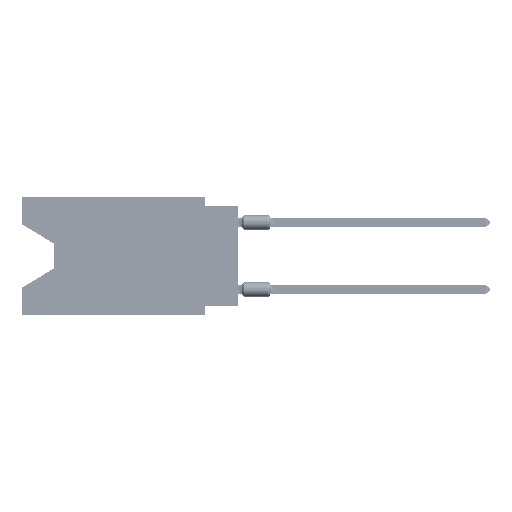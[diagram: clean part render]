
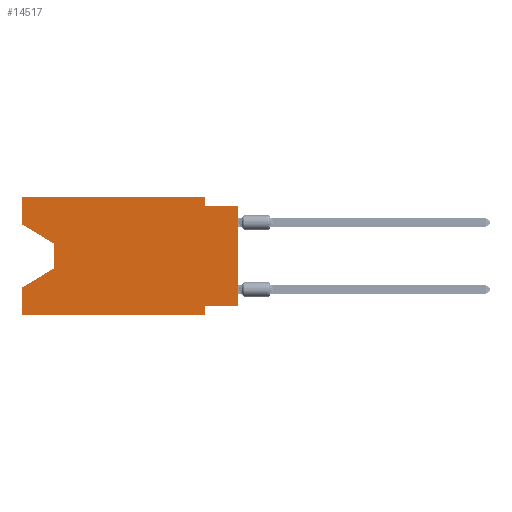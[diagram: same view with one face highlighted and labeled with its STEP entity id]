
A CAD part, left-side view. The second image highlights one B-rep face of the part: STEP entity #14517.
In plain terms, the highlighted planar face has unit normal (-1, 0, 0).
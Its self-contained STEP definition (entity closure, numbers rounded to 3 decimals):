
#1464 = EDGE_LOOP ( 'NONE', ( #14148, #25218, #67241, #67048, #18432, #14422, #58843, #45824, #65367, #66566, #65498, #14328 ) ) ;
#2591 = DIRECTION ( 'NONE',  ( 0., -1., 0. ) ) ;
#3326 = CARTESIAN_POINT ( 'NONE',  ( 0., 16.383, -6.852 ) ) ;
#5219 = VECTOR ( 'NONE', #29691, 1000. ) ;
#6168 = CARTESIAN_POINT ( 'NONE',  ( 0., 16.383, 0. ) ) ;
#6570 = CARTESIAN_POINT ( 'NONE',  ( 0., 13.97, -3.505 ) ) ;
#6710 = CARTESIAN_POINT ( 'NONE',  ( 0., 16.383, 0. ) ) ;
#7194 = DIRECTION ( 'NONE',  ( 0., -0.855, -0.519 ) ) ;
#7883 = CARTESIAN_POINT ( 'NONE',  ( 0., 16.383, -2.038 ) ) ;
#8289 = DIRECTION ( 'NONE',  ( 0., 0.855, -0.519 ) ) ;
#8771 = DIRECTION ( 'NONE',  ( 0., -1., 0. ) ) ;
#8777 = CARTESIAN_POINT ( 'NONE',  ( 0., 13.97, -3.505 ) ) ;
#9254 = CARTESIAN_POINT ( 'NONE',  ( 0., 2.54, -8.89 ) ) ;
#11705 = VECTOR ( 'NONE', #17852, 1000. ) ;
#11786 = CARTESIAN_POINT ( 'NONE',  ( 0., 2.54, 0. ) ) ;
#11862 = EDGE_CURVE ( 'NONE', #12898, #56876, #51616, .T. ) ;
#12177 = DIRECTION ( 'NONE',  ( 0., 0., -1. ) ) ;
#12898 = VERTEX_POINT ( 'NONE', #27450 ) ;
#13046 = CARTESIAN_POINT ( 'NONE',  ( 0., 0., -0.635 ) ) ;
#13644 = VERTEX_POINT ( 'NONE', #22750 ) ;
#14148 = ORIENTED_EDGE ( 'NONE', *, *, #18397, .T. ) ;
#14284 = LINE ( 'NONE', #56065, #5219 ) ;
#14328 = ORIENTED_EDGE ( 'NONE', *, *, #14355, .F. ) ;
#14355 = EDGE_CURVE ( 'NONE', #37788, #39389, #25358, .T. ) ;
#14422 = ORIENTED_EDGE ( 'NONE', *, *, #33079, .F. ) ;
#14517 = ADVANCED_FACE ( 'NONE', ( #53074 ), #16778, .F. ) ;
#15247 = CARTESIAN_POINT ( 'NONE',  ( 0., 16.383, -8.89 ) ) ;
#16778 = PLANE ( 'NONE',  #20786 ) ;
#17025 = VERTEX_POINT ( 'NONE', #35874 ) ;
#17183 = EDGE_CURVE ( 'NONE', #12898, #34606, #53997, .T. ) ;
#17408 = EDGE_CURVE ( 'NONE', #13644, #37928, #62152, .T. ) ;
#17852 = DIRECTION ( 'NONE',  ( 0., -1., 0. ) ) ;
#18132 = LINE ( 'NONE', #28728, #66179 ) ;
#18397 = EDGE_CURVE ( 'NONE', #37788, #43835, #18132, .T. ) ;
#18432 = ORIENTED_EDGE ( 'NONE', *, *, #17408, .T. ) ;
#18843 = VECTOR ( 'NONE', #66294, 1000. ) ;
#20786 = AXIS2_PLACEMENT_3D ( 'NONE', #6168, #53743, #47935 ) ;
#21721 = EDGE_CURVE ( 'NONE', #13644, #65438, #14284, .T. ) ;
#22450 = VERTEX_POINT ( 'NONE', #32568 ) ;
#22750 = CARTESIAN_POINT ( 'NONE',  ( 0., 16.383, -8.89 ) ) ;
#23682 = EDGE_CURVE ( 'NONE', #44118, #17025, #54889, .T. ) ;
#25218 = ORIENTED_EDGE ( 'NONE', *, *, #55387, .T. ) ;
#25358 = LINE ( 'NONE', #36972, #29541 ) ;
#25594 = CARTESIAN_POINT ( 'NONE',  ( 0., 2.54, 0. ) ) ;
#27450 = CARTESIAN_POINT ( 'NONE',  ( 0., 0., -8.255 ) ) ;
#28728 = CARTESIAN_POINT ( 'NONE',  ( 0., 16.383, -2.038 ) ) ;
#29541 = VECTOR ( 'NONE', #36636, 1000. ) ;
#29691 = DIRECTION ( 'NONE',  ( 0., 0., 1. ) ) ;
#30516 = LINE ( 'NONE', #66803, #65300 ) ;
#30754 = CARTESIAN_POINT ( 'NONE',  ( 0., 2.54, -8.255 ) ) ;
#32568 = CARTESIAN_POINT ( 'NONE',  ( 0., 13.97, -5.385 ) ) ;
#33079 = EDGE_CURVE ( 'NONE', #56876, #37928, #58762, .T. ) ;
#33723 = LINE ( 'NONE', #6710, #36625 ) ;
#33768 = DIRECTION ( 'NONE',  ( 0., 0., 1. ) ) ;
#34127 = VECTOR ( 'NONE', #12177, 1000. ) ;
#34606 = VERTEX_POINT ( 'NONE', #38124 ) ;
#35764 = CARTESIAN_POINT ( 'NONE',  ( 0., 16.383, 0. ) ) ;
#35874 = CARTESIAN_POINT ( 'NONE',  ( 0., 2.54, -0.635 ) ) ;
#36625 = VECTOR ( 'NONE', #2591, 1000. ) ;
#36636 = DIRECTION ( 'NONE',  ( 0., 0., 1. ) ) ;
#36972 = CARTESIAN_POINT ( 'NONE',  ( 0., 16.383, 0. ) ) ;
#37788 = VERTEX_POINT ( 'NONE', #7883 ) ;
#37928 = VERTEX_POINT ( 'NONE', #9254 ) ;
#38124 = CARTESIAN_POINT ( 'NONE',  ( 0., 0., -0.635 ) ) ;
#39389 = VERTEX_POINT ( 'NONE', #35764 ) ;
#41468 = VECTOR ( 'NONE', #64486, 1000. ) ;
#41988 = VECTOR ( 'NONE', #8771, 1000. ) ;
#42682 = CARTESIAN_POINT ( 'NONE',  ( 0., 0., -8.255 ) ) ;
#43835 = VERTEX_POINT ( 'NONE', #6570 ) ;
#44118 = VERTEX_POINT ( 'NONE', #25594 ) ;
#45824 = ORIENTED_EDGE ( 'NONE', *, *, #17183, .T. ) ;
#47935 = DIRECTION ( 'NONE',  ( 0., 0., -1. ) ) ;
#49326 = EDGE_CURVE ( 'NONE', #22450, #65438, #30516, .T. ) ;
#49884 = LINE ( 'NONE', #8777, #18843 ) ;
#51616 = LINE ( 'NONE', #42682, #53583 ) ;
#53074 = FACE_OUTER_BOUND ( 'NONE', #1464, .T. ) ;
#53583 = VECTOR ( 'NONE', #63558, 1000. ) ;
#53743 = DIRECTION ( 'NONE',  ( 1., 0., 0. ) ) ;
#53997 = LINE ( 'NONE', #65593, #64893 ) ;
#54889 = LINE ( 'NONE', #11786, #41468 ) ;
#55387 = EDGE_CURVE ( 'NONE', #43835, #22450, #49884, .T. ) ;
#56065 = CARTESIAN_POINT ( 'NONE',  ( 0., 16.383, 0. ) ) ;
#56876 = VERTEX_POINT ( 'NONE', #30754 ) ;
#58762 = LINE ( 'NONE', #59084, #34127 ) ;
#58843 = ORIENTED_EDGE ( 'NONE', *, *, #11862, .F. ) ;
#58897 = EDGE_CURVE ( 'NONE', #39389, #44118, #33723, .T. ) ;
#59084 = CARTESIAN_POINT ( 'NONE',  ( 0., 2.54, -8.89 ) ) ;
#59627 = LINE ( 'NONE', #13046, #11705 ) ;
#62152 = LINE ( 'NONE', #15247, #41988 ) ;
#63187 = EDGE_CURVE ( 'NONE', #17025, #34606, #59627, .T. ) ;
#63558 = DIRECTION ( 'NONE',  ( 0., 1., 0. ) ) ;
#64486 = DIRECTION ( 'NONE',  ( 0., 0., -1. ) ) ;
#64893 = VECTOR ( 'NONE', #33768, 1000. ) ;
#65300 = VECTOR ( 'NONE', #8289, 1000. ) ;
#65367 = ORIENTED_EDGE ( 'NONE', *, *, #63187, .F. ) ;
#65438 = VERTEX_POINT ( 'NONE', #3326 ) ;
#65498 = ORIENTED_EDGE ( 'NONE', *, *, #58897, .F. ) ;
#65593 = CARTESIAN_POINT ( 'NONE',  ( 0., 0., 0. ) ) ;
#66179 = VECTOR ( 'NONE', #7194, 1000. ) ;
#66294 = DIRECTION ( 'NONE',  ( 0., 0., -1. ) ) ;
#66566 = ORIENTED_EDGE ( 'NONE', *, *, #23682, .F. ) ;
#66803 = CARTESIAN_POINT ( 'NONE',  ( 0., 13.97, -5.385 ) ) ;
#67048 = ORIENTED_EDGE ( 'NONE', *, *, #21721, .F. ) ;
#67241 = ORIENTED_EDGE ( 'NONE', *, *, #49326, .T. ) ;
